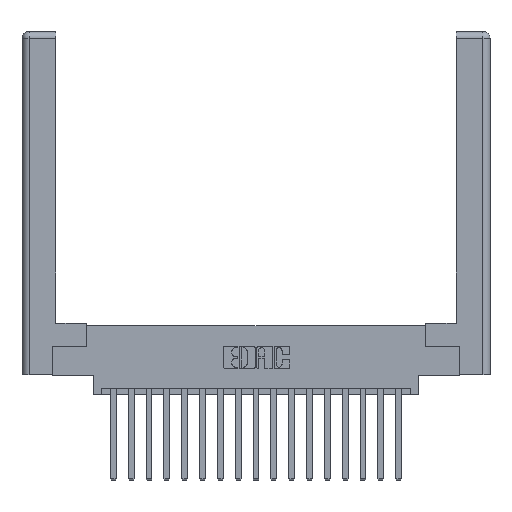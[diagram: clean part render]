
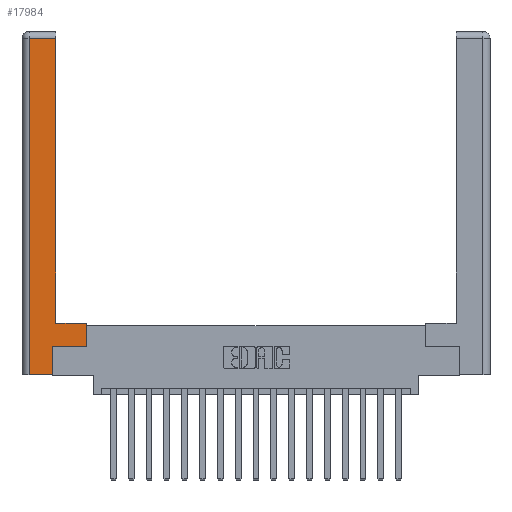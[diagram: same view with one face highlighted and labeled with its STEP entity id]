
A CAD part, top view. The second image highlights one B-rep face of the part: STEP entity #17984.
In plain terms, the highlighted planar face has unit normal (0, 0, 1).
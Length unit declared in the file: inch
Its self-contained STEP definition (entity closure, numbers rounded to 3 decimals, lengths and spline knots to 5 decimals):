
#11 = EDGE_CURVE ( 'NONE', #10871, #1305, #5551, .T. ) ;
#73 = VERTEX_POINT ( 'NONE', #17366 ) ;
#699 = LINE ( 'NONE', #1775, #8713 ) ;
#715 = ORIENTED_EDGE ( 'NONE', *, *, #9689, .T. ) ;
#979 = DIRECTION ( 'NONE',  ( 0., 1., 0. ) ) ;
#1209 = LINE ( 'NONE', #11576, #12020 ) ;
#1305 = VERTEX_POINT ( 'NONE', #15058 ) ;
#1360 = FACE_OUTER_BOUND ( 'NONE', #11386, .T. ) ;
#1580 = VERTEX_POINT ( 'NONE', #10554 ) ;
#1775 = CARTESIAN_POINT ( 'NONE',  ( 0.565, 0.45, 0. ) ) ;
#2000 = CARTESIAN_POINT ( 'NONE',  ( 0.0615, 2.94, 0. ) ) ;
#2119 = CARTESIAN_POINT ( 'NONE',  ( 0.0615, 2.94, 0. ) ) ;
#2333 = VERTEX_POINT ( 'NONE', #3729 ) ;
#2469 = DIRECTION ( 'NONE',  ( 1., 0., 0. ) ) ;
#2692 = VERTEX_POINT ( 'NONE', #15476 ) ;
#3285 = LINE ( 'NONE', #15406, #16638 ) ;
#3528 = LINE ( 'NONE', #9270, #12507 ) ;
#3725 = CARTESIAN_POINT ( 'NONE',  ( 0.295, 3., 0. ) ) ;
#3729 = CARTESIAN_POINT ( 'NONE',  ( 0.265, 0., 0. ) ) ;
#4675 = CARTESIAN_POINT ( 'NONE',  ( 0.265, 0.245, 0. ) ) ;
#4820 = LINE ( 'NONE', #2119, #14691 ) ;
#4878 = CARTESIAN_POINT ( 'NONE',  ( 0., 0., 0. ) ) ;
#5119 = VERTEX_POINT ( 'NONE', #4675 ) ;
#5446 = ORIENTED_EDGE ( 'NONE', *, *, #10154, .T. ) ;
#5479 = VERTEX_POINT ( 'NONE', #2000 ) ;
#5551 = LINE ( 'NONE', #3725, #18874 ) ;
#6615 = ORIENTED_EDGE ( 'NONE', *, *, #7427, .T. ) ;
#7062 = VECTOR ( 'NONE', #16497, 39.37008 ) ;
#7427 = EDGE_CURVE ( 'NONE', #2333, #5119, #13034, .T. ) ;
#8550 = DIRECTION ( 'NONE',  ( 0., -1., 0. ) ) ;
#8713 = VECTOR ( 'NONE', #979, 39.37008 ) ;
#8892 = AXIS2_PLACEMENT_3D ( 'NONE', #4878, #12272, #16727 ) ;
#9025 = CARTESIAN_POINT ( 'NONE',  ( 0.265, 0.245, 0. ) ) ;
#9210 = DIRECTION ( 'NONE',  ( -1., 0., 0. ) ) ;
#9270 = CARTESIAN_POINT ( 'NONE',  ( 0.295, 0.45, 0. ) ) ;
#9385 = ORIENTED_EDGE ( 'NONE', *, *, #9785, .T. ) ;
#9436 = PLANE ( 'NONE',  #8892 ) ;
#9679 = ORIENTED_EDGE ( 'NONE', *, *, #10017, .T. ) ;
#9689 = EDGE_CURVE ( 'NONE', #1580, #10871, #3528, .T. ) ;
#9785 = EDGE_CURVE ( 'NONE', #2692, #2333, #3285, .T. ) ;
#10017 = EDGE_CURVE ( 'NONE', #5479, #2692, #1209, .T. ) ;
#10154 = EDGE_CURVE ( 'NONE', #5119, #73, #11783, .T. ) ;
#10554 = CARTESIAN_POINT ( 'NONE',  ( 0.565, 0.45, 0. ) ) ;
#10871 = VERTEX_POINT ( 'NONE', #15632 ) ;
#11292 = ORIENTED_EDGE ( 'NONE', *, *, #14626, .T. ) ;
#11386 = EDGE_LOOP ( 'NONE', ( #13257, #14106, #9679, #9385, #6615, #5446, #11292, #715 ) ) ;
#11576 = CARTESIAN_POINT ( 'NONE',  ( 0.0615, 0., 0. ) ) ;
#11783 = LINE ( 'NONE', #11843, #15240 ) ;
#11843 = CARTESIAN_POINT ( 'NONE',  ( 0.565, 0.245, 0. ) ) ;
#12020 = VECTOR ( 'NONE', #8550, 39.37008 ) ;
#12272 = DIRECTION ( 'NONE',  ( 0., 0., -1. ) ) ;
#12507 = VECTOR ( 'NONE', #9210, 39.37008 ) ;
#13034 = LINE ( 'NONE', #9025, #7062 ) ;
#13257 = ORIENTED_EDGE ( 'NONE', *, *, #11, .T. ) ;
#13670 = DIRECTION ( 'NONE',  ( -1., 0., 0. ) ) ;
#13994 = DIRECTION ( 'NONE',  ( 0., 1., 0. ) ) ;
#14106 = ORIENTED_EDGE ( 'NONE', *, *, #18002, .T. ) ;
#14626 = EDGE_CURVE ( 'NONE', #73, #1580, #699, .T. ) ;
#14691 = VECTOR ( 'NONE', #13670, 39.37008 ) ;
#15058 = CARTESIAN_POINT ( 'NONE',  ( 0.295, 2.94, 0. ) ) ;
#15240 = VECTOR ( 'NONE', #17780, 39.37008 ) ;
#15406 = CARTESIAN_POINT ( 'NONE',  ( 0.265, 0., 0. ) ) ;
#15476 = CARTESIAN_POINT ( 'NONE',  ( 0.0615, 0., 0. ) ) ;
#15632 = CARTESIAN_POINT ( 'NONE',  ( 0.295, 0.45, 0. ) ) ;
#16497 = DIRECTION ( 'NONE',  ( 0., 1., 0. ) ) ;
#16638 = VECTOR ( 'NONE', #2469, 39.37008 ) ;
#16727 = DIRECTION ( 'NONE',  ( -1., 0., 0. ) ) ;
#17366 = CARTESIAN_POINT ( 'NONE',  ( 0.565, 0.245, 0. ) ) ;
#17780 = DIRECTION ( 'NONE',  ( 1., 0., 0. ) ) ;
#17984 = ADVANCED_FACE ( 'NONE', ( #1360 ), #9436, .F. ) ;
#18002 = EDGE_CURVE ( 'NONE', #1305, #5479, #4820, .T. ) ;
#18874 = VECTOR ( 'NONE', #13994, 39.37008 ) ;
